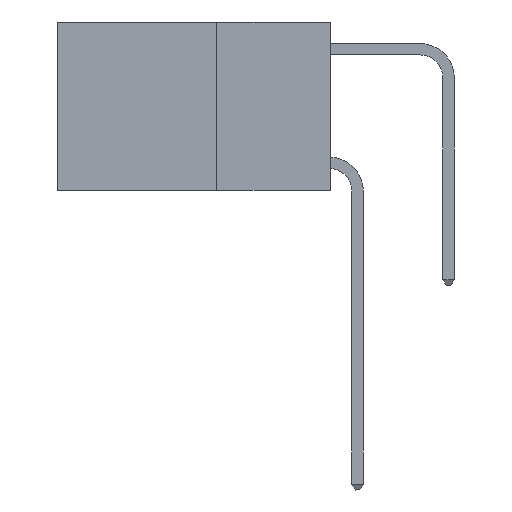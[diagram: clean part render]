
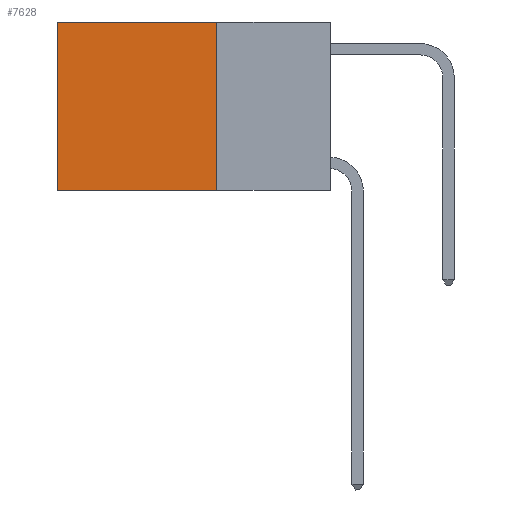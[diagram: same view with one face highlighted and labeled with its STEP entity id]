
A CAD part, left-side view. The second image highlights one B-rep face of the part: STEP entity #7628.
In plain terms, the highlighted planar face has unit normal (-1, 0, 0).
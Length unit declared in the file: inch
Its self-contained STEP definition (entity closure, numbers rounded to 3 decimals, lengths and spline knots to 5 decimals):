
#141 = DIRECTION ( 'NONE',  ( 1., 0., 0. ) ) ;
#494 = CARTESIAN_POINT ( 'NONE',  ( 0.2625, 0.25, 0. ) ) ;
#784 = VECTOR ( 'NONE', #1120, 39.37008 ) ;
#1120 = DIRECTION ( 'NONE',  ( 0., 0., -1. ) ) ;
#2355 = CARTESIAN_POINT ( 'NONE',  ( 0.2625, 0.6, 0. ) ) ;
#2627 = LINE ( 'NONE', #8626, #7921 ) ;
#2889 = CARTESIAN_POINT ( 'NONE',  ( 0.2625, 0.6, -0.37 ) ) ;
#3551 = ORIENTED_EDGE ( 'NONE', *, *, #9057, .F. ) ;
#3632 = FACE_OUTER_BOUND ( 'NONE', #10654, .T. ) ;
#4027 = VECTOR ( 'NONE', #8673, 39.37008 ) ;
#4345 = PLANE ( 'NONE',  #9174 ) ;
#4639 = VERTEX_POINT ( 'NONE', #8574 ) ;
#5771 = VERTEX_POINT ( 'NONE', #2355 ) ;
#6155 = DIRECTION ( 'NONE',  ( 0., 1., 0. ) ) ;
#6904 = CARTESIAN_POINT ( 'NONE',  ( 0.2625, 0.25, 0. ) ) ;
#7579 = EDGE_CURVE ( 'NONE', #10140, #8221, #2627, .T. ) ;
#7628 = ADVANCED_FACE ( 'NONE', ( #3632 ), #4345, .F. ) ;
#7693 = LINE ( 'NONE', #6904, #10805 ) ;
#7778 = CARTESIAN_POINT ( 'NONE',  ( 0.2625, 0.25, 0. ) ) ;
#7921 = VECTOR ( 'NONE', #10467, 39.37008 ) ;
#8221 = VERTEX_POINT ( 'NONE', #2889 ) ;
#8255 = ORIENTED_EDGE ( 'NONE', *, *, #10220, .T. ) ;
#8484 = EDGE_CURVE ( 'NONE', #4639, #5771, #7693, .T. ) ;
#8574 = CARTESIAN_POINT ( 'NONE',  ( 0.2625, 0.25, 0. ) ) ;
#8626 = CARTESIAN_POINT ( 'NONE',  ( 0.2625, 0.25, -0.37 ) ) ;
#8673 = DIRECTION ( 'NONE',  ( 0., 0., -1. ) ) ;
#8737 = DIRECTION ( 'NONE',  ( 0., 0., -1. ) ) ;
#8924 = LINE ( 'NONE', #494, #784 ) ;
#8997 = ORIENTED_EDGE ( 'NONE', *, *, #7579, .F. ) ;
#9057 = EDGE_CURVE ( 'NONE', #4639, #10140, #8924, .T. ) ;
#9174 = AXIS2_PLACEMENT_3D ( 'NONE', #7778, #141, #8737 ) ;
#10140 = VERTEX_POINT ( 'NONE', #10803 ) ;
#10192 = ORIENTED_EDGE ( 'NONE', *, *, #8484, .T. ) ;
#10220 = EDGE_CURVE ( 'NONE', #5771, #8221, #11076, .T. ) ;
#10232 = CARTESIAN_POINT ( 'NONE',  ( 0.2625, 0.6, 0. ) ) ;
#10467 = DIRECTION ( 'NONE',  ( 0., 1., 0. ) ) ;
#10654 = EDGE_LOOP ( 'NONE', ( #8255, #8997, #3551, #10192 ) ) ;
#10803 = CARTESIAN_POINT ( 'NONE',  ( 0.2625, 0.25, -0.37 ) ) ;
#10805 = VECTOR ( 'NONE', #6155, 39.37008 ) ;
#11076 = LINE ( 'NONE', #10232, #4027 ) ;
